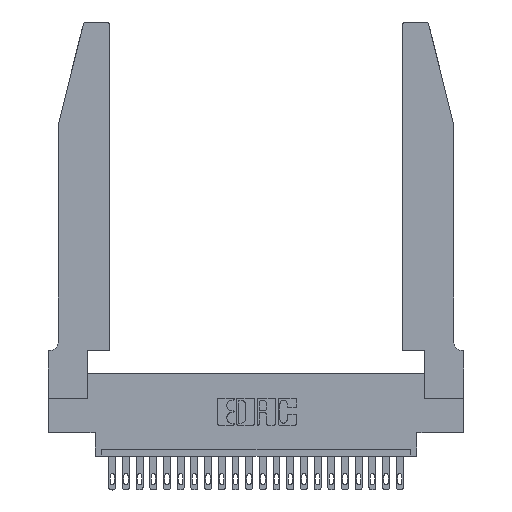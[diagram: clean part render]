
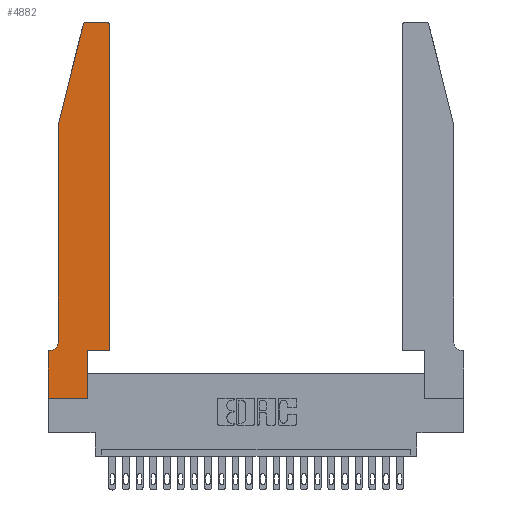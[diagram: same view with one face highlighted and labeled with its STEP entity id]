
A CAD part, top view. The second image highlights one B-rep face of the part: STEP entity #4882.
In plain terms, the highlighted planar face has unit normal (0, 0, 1).
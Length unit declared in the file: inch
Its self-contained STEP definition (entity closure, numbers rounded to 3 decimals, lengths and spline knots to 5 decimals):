
#264 = VERTEX_POINT ( 'NONE', #14408 ) ;
#408 = CIRCLE ( 'NONE', #12228, 0.03 ) ;
#1923 = LINE ( 'NONE', #17037, #6891 ) ;
#3291 = VECTOR ( 'NONE', #17734, 39.37008 ) ;
#3554 = EDGE_CURVE ( 'NONE', #20596, #21385, #3761, .T. ) ;
#3611 = PLANE ( 'NONE',  #20349 ) ;
#3761 = LINE ( 'NONE', #12765, #9552 ) ;
#4661 = CARTESIAN_POINT ( 'NONE',  ( 0.25487, 2.72718, 0.37 ) ) ;
#4882 = ADVANCED_FACE ( 'NONE', ( #8933 ), #3611, .T. ) ;
#5065 = DIRECTION ( 'NONE',  ( -1., 0., 0. ) ) ;
#5103 = ORIENTED_EDGE ( 'NONE', *, *, #10109, .T. ) ;
#5120 = ORIENTED_EDGE ( 'NONE', *, *, #5405, .T. ) ;
#5137 = CARTESIAN_POINT ( 'NONE',  ( 0.2865, 0., 0.37 ) ) ;
#5405 = EDGE_CURVE ( 'NONE', #23911, #12315, #19647, .T. ) ;
#5558 = DIRECTION ( 'NONE',  ( -1., 0., 0. ) ) ;
#5688 = DIRECTION ( 'NONE',  ( 1., 0., 0. ) ) ;
#6239 = LINE ( 'NONE', #7246, #20462 ) ;
#6293 = CIRCLE ( 'NONE', #16191, 0.07 ) ;
#6424 = EDGE_CURVE ( 'NONE', #12863, #20586, #7513, .T. ) ;
#6429 = ORIENTED_EDGE ( 'NONE', *, *, #9264, .T. ) ;
#6707 = EDGE_LOOP ( 'NONE', ( #9200, #7201, #9135, #13278, #12608, #16312, #12182, #12698, #5120, #10027, #6429, #5103 ) ) ;
#6891 = VECTOR ( 'NONE', #12714, 39.37008 ) ;
#7201 = ORIENTED_EDGE ( 'NONE', *, *, #16562, .T. ) ;
#7246 = CARTESIAN_POINT ( 'NONE',  ( 0.4505, 0.35, 0.37 ) ) ;
#7459 = CARTESIAN_POINT ( 'NONE',  ( 0.0755, 0.35, 0.37 ) ) ;
#7478 = DIRECTION ( 'NONE',  ( 1., 0., 0. ) ) ;
#7513 = LINE ( 'NONE', #7567, #8971 ) ;
#7567 = CARTESIAN_POINT ( 'NONE',  ( 0.0755, 2., 0.37 ) ) ;
#7862 = VECTOR ( 'NONE', #12723, 39.37008 ) ;
#7867 = DIRECTION ( 'NONE',  ( 0., 1., 0. ) ) ;
#7945 = CARTESIAN_POINT ( 'NONE',  ( 0., 0., 0.37 ) ) ;
#8163 = EDGE_CURVE ( 'NONE', #264, #12418, #6293, .T. ) ;
#8195 = CARTESIAN_POINT ( 'NONE',  ( 0.4205, 2.72, 0.37 ) ) ;
#8272 = EDGE_CURVE ( 'NONE', #12315, #8924, #1923, .T. ) ;
#8335 = CARTESIAN_POINT ( 'NONE',  ( 0.284, 2.75, 0.37 ) ) ;
#8367 = DIRECTION ( 'NONE',  ( 0., 0., 1. ) ) ;
#8667 = CARTESIAN_POINT ( 'NONE',  ( 0.0755, 2., 0.37 ) ) ;
#8924 = VERTEX_POINT ( 'NONE', #12267 ) ;
#8933 = FACE_OUTER_BOUND ( 'NONE', #6707, .T. ) ;
#8971 = VECTOR ( 'NONE', #13769, 39.37008 ) ;
#9135 = ORIENTED_EDGE ( 'NONE', *, *, #6424, .T. ) ;
#9200 = ORIENTED_EDGE ( 'NONE', *, *, #3554, .T. ) ;
#9264 = EDGE_CURVE ( 'NONE', #8924, #18069, #6239, .T. ) ;
#9552 = VECTOR ( 'NONE', #5558, 39.37008 ) ;
#9764 = VECTOR ( 'NONE', #7867, 39.37008 ) ;
#10027 = ORIENTED_EDGE ( 'NONE', *, *, #8272, .T. ) ;
#10109 = EDGE_CURVE ( 'NONE', #18069, #20596, #22762, .T. ) ;
#10589 = CARTESIAN_POINT ( 'NONE',  ( 0., 0.35, 0.37 ) ) ;
#10763 = EDGE_CURVE ( 'NONE', #20151, #23911, #19807, .T. ) ;
#10954 = DIRECTION ( 'NONE',  ( 0., 0., -1. ) ) ;
#11146 = CARTESIAN_POINT ( 'NONE',  ( 0.2865, 0.35, 0.37 ) ) ;
#11193 = CARTESIAN_POINT ( 'NONE',  ( 0.0055, 0.42, 0.37 ) ) ;
#11472 = CARTESIAN_POINT ( 'NONE',  ( 0.4205, 2.75, 0.37 ) ) ;
#11942 = VECTOR ( 'NONE', #15406, 39.37008 ) ;
#12182 = ORIENTED_EDGE ( 'NONE', *, *, #22389, .T. ) ;
#12228 = AXIS2_PLACEMENT_3D ( 'NONE', #20131, #20213, #5688 ) ;
#12267 = CARTESIAN_POINT ( 'NONE',  ( 0.4505, 0.35, 0.37 ) ) ;
#12315 = VERTEX_POINT ( 'NONE', #11146 ) ;
#12418 = VERTEX_POINT ( 'NONE', #13642 ) ;
#12608 = ORIENTED_EDGE ( 'NONE', *, *, #8163, .T. ) ;
#12698 = ORIENTED_EDGE ( 'NONE', *, *, #10763, .T. ) ;
#12714 = DIRECTION ( 'NONE',  ( 1., 0., 0. ) ) ;
#12723 = DIRECTION ( 'NONE',  ( -1., 0., 0. ) ) ;
#12765 = CARTESIAN_POINT ( 'NONE',  ( 0.2605, 2.75, 0.37 ) ) ;
#12785 = LINE ( 'NONE', #7459, #7862 ) ;
#12863 = VERTEX_POINT ( 'NONE', #4661 ) ;
#13278 = ORIENTED_EDGE ( 'NONE', *, *, #19042, .T. ) ;
#13491 = CARTESIAN_POINT ( 'NONE',  ( 0., 0., 0.37 ) ) ;
#13642 = CARTESIAN_POINT ( 'NONE',  ( 0.0055, 0.35, 0.37 ) ) ;
#13769 = DIRECTION ( 'NONE',  ( -0.239, -0.971, 0. ) ) ;
#14408 = CARTESIAN_POINT ( 'NONE',  ( 0.0755, 0.42, 0.37 ) ) ;
#15406 = DIRECTION ( 'NONE',  ( 1., 0., 0. ) ) ;
#16191 = AXIS2_PLACEMENT_3D ( 'NONE', #11193, #10954, #5065 ) ;
#16312 = ORIENTED_EDGE ( 'NONE', *, *, #19777, .T. ) ;
#16562 = EDGE_CURVE ( 'NONE', #21385, #12863, #408, .T. ) ;
#16563 = DIRECTION ( 'NONE',  ( 0., 0., 1. ) ) ;
#16710 = VECTOR ( 'NONE', #21049, 39.37008 ) ;
#17037 = CARTESIAN_POINT ( 'NONE',  ( 0.4505, 0.35, 0.37 ) ) ;
#17234 = VERTEX_POINT ( 'NONE', #10589 ) ;
#17734 = DIRECTION ( 'NONE',  ( 0., -1., 0. ) ) ;
#18069 = VERTEX_POINT ( 'NONE', #21050 ) ;
#18521 = CARTESIAN_POINT ( 'NONE',  ( 0., 0.35, 0.37 ) ) ;
#18978 = CARTESIAN_POINT ( 'NONE',  ( 0.2865, 0.35, 0.37 ) ) ;
#19023 = CARTESIAN_POINT ( 'NONE',  ( 0.0755, 2., 0.37 ) ) ;
#19042 = EDGE_CURVE ( 'NONE', #20586, #264, #21296, .T. ) ;
#19647 = LINE ( 'NONE', #18978, #9764 ) ;
#19777 = EDGE_CURVE ( 'NONE', #12418, #17234, #12785, .T. ) ;
#19807 = LINE ( 'NONE', #13491, #11942 ) ;
#20131 = CARTESIAN_POINT ( 'NONE',  ( 0.284, 2.72, 0.37 ) ) ;
#20151 = VERTEX_POINT ( 'NONE', #23144 ) ;
#20208 = DIRECTION ( 'NONE',  ( 0., 1., 0. ) ) ;
#20213 = DIRECTION ( 'NONE',  ( 0., 0., 1. ) ) ;
#20349 = AXIS2_PLACEMENT_3D ( 'NONE', #18521, #16563, #7478 ) ;
#20462 = VECTOR ( 'NONE', #20208, 39.37008 ) ;
#20586 = VERTEX_POINT ( 'NONE', #19023 ) ;
#20596 = VERTEX_POINT ( 'NONE', #11472 ) ;
#21049 = DIRECTION ( 'NONE',  ( 0., -1., 0. ) ) ;
#21050 = CARTESIAN_POINT ( 'NONE',  ( 0.4505, 2.72, 0.37 ) ) ;
#21296 = LINE ( 'NONE', #8667, #3291 ) ;
#21358 = DIRECTION ( 'NONE',  ( 1., 0., 0. ) ) ;
#21385 = VERTEX_POINT ( 'NONE', #8335 ) ;
#21807 = AXIS2_PLACEMENT_3D ( 'NONE', #8195, #8367, #21358 ) ;
#22389 = EDGE_CURVE ( 'NONE', #17234, #20151, #23731, .T. ) ;
#22762 = CIRCLE ( 'NONE', #21807, 0.03 ) ;
#23144 = CARTESIAN_POINT ( 'NONE',  ( 0., 0., 0.37 ) ) ;
#23731 = LINE ( 'NONE', #7945, #16710 ) ;
#23911 = VERTEX_POINT ( 'NONE', #5137 ) ;
